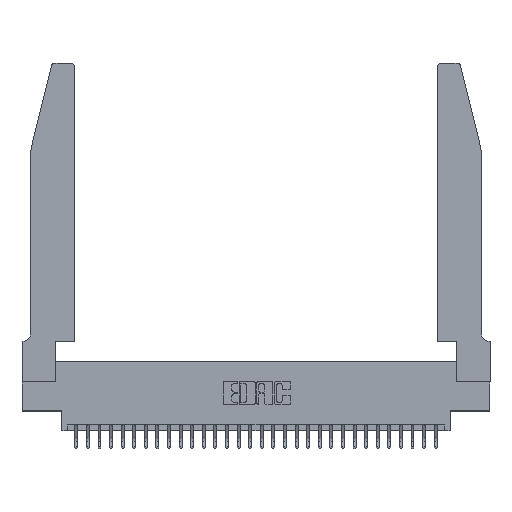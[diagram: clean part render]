
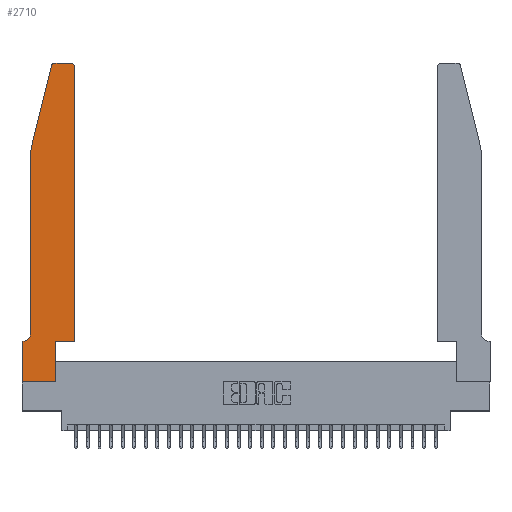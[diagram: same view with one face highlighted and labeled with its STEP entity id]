
A CAD part, top view. The second image highlights one B-rep face of the part: STEP entity #2710.
In plain terms, the highlighted planar face has unit normal (0, 0, 1).
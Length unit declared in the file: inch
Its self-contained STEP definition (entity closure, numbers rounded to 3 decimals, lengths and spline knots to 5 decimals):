
#229 = EDGE_CURVE ( 'NONE', #11222, #1582, #7357, .T. ) ;
#451 = LINE ( 'NONE', #30296, #5070 ) ;
#1128 = VECTOR ( 'NONE', #22046, 39.37008 ) ;
#1489 = DIRECTION ( 'NONE',  ( 1., 0., 0. ) ) ;
#1582 = VERTEX_POINT ( 'NONE', #21165 ) ;
#1690 = ORIENTED_EDGE ( 'NONE', *, *, #1996, .T. ) ;
#1803 = AXIS2_PLACEMENT_3D ( 'NONE', #18896, #26407, #9542 ) ;
#1996 = EDGE_CURVE ( 'NONE', #1582, #22769, #15216, .T. ) ;
#2231 = CIRCLE ( 'NONE', #10768, 0.07 ) ;
#2255 = VERTEX_POINT ( 'NONE', #21249 ) ;
#2285 = EDGE_CURVE ( 'NONE', #29670, #22594, #2231, .T. ) ;
#2710 = ADVANCED_FACE ( 'NONE', ( #15154 ), #23253, .T. ) ;
#3660 = EDGE_LOOP ( 'NONE', ( #6773, #4508, #1690, #21760, #24074, #15107, #5125, #26164, #23659, #28709, #6419, #16576 ) ) ;
#3895 = CARTESIAN_POINT ( 'NONE',  ( 0.0055, 0.42, 0.37 ) ) ;
#4107 = EDGE_CURVE ( 'NONE', #6330, #13605, #6726, .T. ) ;
#4201 = CARTESIAN_POINT ( 'NONE',  ( 0.0755, 2., 0.37 ) ) ;
#4508 = ORIENTED_EDGE ( 'NONE', *, *, #229, .T. ) ;
#5070 = VECTOR ( 'NONE', #23454, 39.37008 ) ;
#5125 = ORIENTED_EDGE ( 'NONE', *, *, #27570, .T. ) ;
#6330 = VERTEX_POINT ( 'NONE', #29921 ) ;
#6419 = ORIENTED_EDGE ( 'NONE', *, *, #4107, .T. ) ;
#6466 = CARTESIAN_POINT ( 'NONE',  ( 0.0755, 0.42, 0.37 ) ) ;
#6546 = DIRECTION ( 'NONE',  ( 1., 0., 0. ) ) ;
#6726 = LINE ( 'NONE', #17637, #27983 ) ;
#6773 = ORIENTED_EDGE ( 'NONE', *, *, #12203, .T. ) ;
#6794 = EDGE_CURVE ( 'NONE', #15173, #6330, #18412, .T. ) ;
#6820 = DIRECTION ( 'NONE',  ( 1., 0., 0. ) ) ;
#7357 = CIRCLE ( 'NONE', #19693, 0.03 ) ;
#7621 = LINE ( 'NONE', #21941, #1128 ) ;
#8630 = CARTESIAN_POINT ( 'NONE',  ( 0., 0., 0.37 ) ) ;
#9015 = DIRECTION ( 'NONE',  ( 0., 0., -1. ) ) ;
#9138 = DIRECTION ( 'NONE',  ( -1., 0., 0. ) ) ;
#9542 = DIRECTION ( 'NONE',  ( 1., 0., 0. ) ) ;
#9650 = DIRECTION ( 'NONE',  ( 0., 0., 1. ) ) ;
#10088 = VECTOR ( 'NONE', #6820, 39.37008 ) ;
#10136 = VERTEX_POINT ( 'NONE', #12946 ) ;
#10768 = AXIS2_PLACEMENT_3D ( 'NONE', #3895, #9015, #14305 ) ;
#10830 = LINE ( 'NONE', #11500, #27544 ) ;
#11173 = EDGE_CURVE ( 'NONE', #22594, #2255, #7621, .T. ) ;
#11222 = VERTEX_POINT ( 'NONE', #15043 ) ;
#11500 = CARTESIAN_POINT ( 'NONE',  ( 0.2865, 0.35, 0.37 ) ) ;
#11608 = DIRECTION ( 'NONE',  ( 0., 1., 0. ) ) ;
#11932 = VECTOR ( 'NONE', #6546, 39.37008 ) ;
#12203 = EDGE_CURVE ( 'NONE', #31543, #11222, #24308, .T. ) ;
#12946 = CARTESIAN_POINT ( 'NONE',  ( 0., 0., 0.37 ) ) ;
#12984 = VERTEX_POINT ( 'NONE', #30179 ) ;
#13300 = VECTOR ( 'NONE', #9138, 39.37008 ) ;
#13374 = CARTESIAN_POINT ( 'NONE',  ( 0.4505, 2.72, 0.37 ) ) ;
#13605 = VERTEX_POINT ( 'NONE', #13374 ) ;
#13888 = LINE ( 'NONE', #8630, #10088 ) ;
#14027 = CARTESIAN_POINT ( 'NONE',  ( 0.4205, 2.75, 0.37 ) ) ;
#14305 = DIRECTION ( 'NONE',  ( -1., 0., 0. ) ) ;
#14868 = CIRCLE ( 'NONE', #22832, 0.03 ) ;
#15043 = CARTESIAN_POINT ( 'NONE',  ( 0.284, 2.75, 0.37 ) ) ;
#15107 = ORIENTED_EDGE ( 'NONE', *, *, #11173, .T. ) ;
#15154 = FACE_OUTER_BOUND ( 'NONE', #3660, .T. ) ;
#15173 = VERTEX_POINT ( 'NONE', #20996 ) ;
#15216 = LINE ( 'NONE', #4201, #29294 ) ;
#15638 = CARTESIAN_POINT ( 'NONE',  ( 0.4505, 0.35, 0.37 ) ) ;
#16576 = ORIENTED_EDGE ( 'NONE', *, *, #18928, .T. ) ;
#17637 = CARTESIAN_POINT ( 'NONE',  ( 0.4505, 0.35, 0.37 ) ) ;
#18145 = CARTESIAN_POINT ( 'NONE',  ( 0.0055, 0.35, 0.37 ) ) ;
#18361 = DIRECTION ( 'NONE',  ( 0., 1., 0. ) ) ;
#18412 = LINE ( 'NONE', #15638, #11932 ) ;
#18896 = CARTESIAN_POINT ( 'NONE',  ( 0., 0.35, 0.37 ) ) ;
#18928 = EDGE_CURVE ( 'NONE', #13605, #31543, #14868, .T. ) ;
#19693 = AXIS2_PLACEMENT_3D ( 'NONE', #23299, #20835, #1489 ) ;
#20768 = DIRECTION ( 'NONE',  ( 0., -1., 0. ) ) ;
#20835 = DIRECTION ( 'NONE',  ( 0., 0., 1. ) ) ;
#20927 = CARTESIAN_POINT ( 'NONE',  ( 0.2605, 2.75, 0.37 ) ) ;
#20996 = CARTESIAN_POINT ( 'NONE',  ( 0.2865, 0.35, 0.37 ) ) ;
#21165 = CARTESIAN_POINT ( 'NONE',  ( 0.25487, 2.72718, 0.37 ) ) ;
#21249 = CARTESIAN_POINT ( 'NONE',  ( 0., 0.35, 0.37 ) ) ;
#21760 = ORIENTED_EDGE ( 'NONE', *, *, #24753, .T. ) ;
#21941 = CARTESIAN_POINT ( 'NONE',  ( 0.0755, 0.35, 0.37 ) ) ;
#22046 = DIRECTION ( 'NONE',  ( -1., 0., 0. ) ) ;
#22594 = VERTEX_POINT ( 'NONE', #18145 ) ;
#22763 = LINE ( 'NONE', #25228, #31171 ) ;
#22769 = VERTEX_POINT ( 'NONE', #29172 ) ;
#22832 = AXIS2_PLACEMENT_3D ( 'NONE', #24175, #9650, #26618 ) ;
#23253 = PLANE ( 'NONE',  #1803 ) ;
#23299 = CARTESIAN_POINT ( 'NONE',  ( 0.284, 2.72, 0.37 ) ) ;
#23318 = EDGE_CURVE ( 'NONE', #12984, #15173, #10830, .T. ) ;
#23454 = DIRECTION ( 'NONE',  ( 0., -1., 0. ) ) ;
#23659 = ORIENTED_EDGE ( 'NONE', *, *, #23318, .T. ) ;
#24074 = ORIENTED_EDGE ( 'NONE', *, *, #2285, .T. ) ;
#24175 = CARTESIAN_POINT ( 'NONE',  ( 0.4205, 2.72, 0.37 ) ) ;
#24308 = LINE ( 'NONE', #20927, #13300 ) ;
#24753 = EDGE_CURVE ( 'NONE', #22769, #29670, #22763, .T. ) ;
#25228 = CARTESIAN_POINT ( 'NONE',  ( 0.0755, 2., 0.37 ) ) ;
#26164 = ORIENTED_EDGE ( 'NONE', *, *, #26982, .T. ) ;
#26407 = DIRECTION ( 'NONE',  ( 0., 0., 1. ) ) ;
#26618 = DIRECTION ( 'NONE',  ( 1., 0., 0. ) ) ;
#26982 = EDGE_CURVE ( 'NONE', #10136, #12984, #13888, .T. ) ;
#27544 = VECTOR ( 'NONE', #11608, 39.37008 ) ;
#27570 = EDGE_CURVE ( 'NONE', #2255, #10136, #451, .T. ) ;
#27983 = VECTOR ( 'NONE', #18361, 39.37008 ) ;
#28434 = DIRECTION ( 'NONE',  ( -0.239, -0.971, 0. ) ) ;
#28709 = ORIENTED_EDGE ( 'NONE', *, *, #6794, .T. ) ;
#29172 = CARTESIAN_POINT ( 'NONE',  ( 0.0755, 2., 0.37 ) ) ;
#29294 = VECTOR ( 'NONE', #28434, 39.37008 ) ;
#29670 = VERTEX_POINT ( 'NONE', #6466 ) ;
#29921 = CARTESIAN_POINT ( 'NONE',  ( 0.4505, 0.35, 0.37 ) ) ;
#30179 = CARTESIAN_POINT ( 'NONE',  ( 0.2865, 0., 0.37 ) ) ;
#30296 = CARTESIAN_POINT ( 'NONE',  ( 0., 0., 0.37 ) ) ;
#31171 = VECTOR ( 'NONE', #20768, 39.37008 ) ;
#31543 = VERTEX_POINT ( 'NONE', #14027 ) ;
